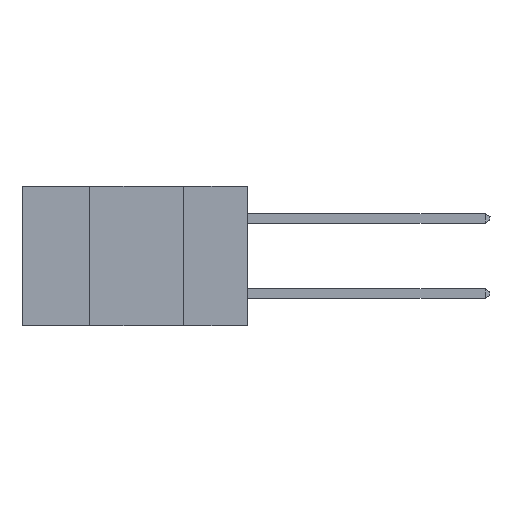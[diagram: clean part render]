
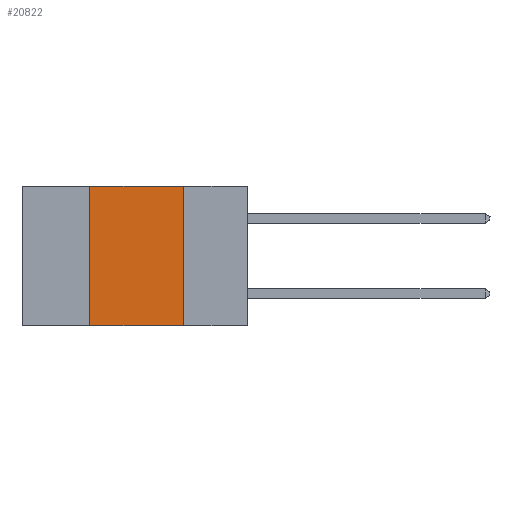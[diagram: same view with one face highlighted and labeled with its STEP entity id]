
A CAD part, left-side view. The second image highlights one B-rep face of the part: STEP entity #20822.
In plain terms, the highlighted planar face has unit normal (-1, 0, 0).
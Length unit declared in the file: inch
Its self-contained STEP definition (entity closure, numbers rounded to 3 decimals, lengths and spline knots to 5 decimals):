
#309 = VERTEX_POINT ( 'NONE', #16970 ) ;
#431 = LINE ( 'NONE', #25511, #8596 ) ;
#1226 = ORIENTED_EDGE ( 'NONE', *, *, #17684, .F. ) ;
#1428 = EDGE_LOOP ( 'NONE', ( #19657, #1226, #23308, #25156 ) ) ;
#2386 = DIRECTION ( 'NONE',  ( 0., -1., 0. ) ) ;
#2614 = VECTOR ( 'NONE', #24374, 39.37008 ) ;
#3199 = CARTESIAN_POINT ( 'NONE',  ( 0., 0.42, -0.37 ) ) ;
#4906 = LINE ( 'NONE', #6582, #13928 ) ;
#5536 = CARTESIAN_POINT ( 'NONE',  ( 0., 0.42, 0. ) ) ;
#6017 = VECTOR ( 'NONE', #7175, 39.37008 ) ;
#6582 = CARTESIAN_POINT ( 'NONE',  ( 0., 0.6, 0. ) ) ;
#6788 = VERTEX_POINT ( 'NONE', #23027 ) ;
#7175 = DIRECTION ( 'NONE',  ( 0., 0., -1. ) ) ;
#8028 = EDGE_CURVE ( 'NONE', #309, #6788, #13015, .T. ) ;
#8596 = VECTOR ( 'NONE', #2386, 39.37008 ) ;
#9742 = PLANE ( 'NONE',  #25899 ) ;
#12132 = EDGE_CURVE ( 'NONE', #26871, #19984, #13759, .T. ) ;
#13015 = LINE ( 'NONE', #15361, #6017 ) ;
#13416 = DIRECTION ( 'NONE',  ( 1., 0., 0. ) ) ;
#13759 = LINE ( 'NONE', #3199, #2614 ) ;
#13928 = VECTOR ( 'NONE', #19714, 39.37008 ) ;
#15361 = CARTESIAN_POINT ( 'NONE',  ( 0., 0.17, -0.37 ) ) ;
#15471 = FACE_OUTER_BOUND ( 'NONE', #1428, .T. ) ;
#16970 = CARTESIAN_POINT ( 'NONE',  ( 0., 0.17, 0. ) ) ;
#17684 = EDGE_CURVE ( 'NONE', #19984, #309, #4906, .T. ) ;
#18196 = CARTESIAN_POINT ( 'NONE',  ( 0., 0.6, 0. ) ) ;
#19657 = ORIENTED_EDGE ( 'NONE', *, *, #8028, .F. ) ;
#19714 = DIRECTION ( 'NONE',  ( 0., -1., 0. ) ) ;
#19737 = EDGE_CURVE ( 'NONE', #26871, #6788, #431, .T. ) ;
#19984 = VERTEX_POINT ( 'NONE', #5536 ) ;
#20453 = CARTESIAN_POINT ( 'NONE',  ( 0., 0.42, -0.37 ) ) ;
#20822 = ADVANCED_FACE ( 'NONE', ( #15471 ), #9742, .F. ) ;
#23027 = CARTESIAN_POINT ( 'NONE',  ( 0., 0.17, -0.37 ) ) ;
#23308 = ORIENTED_EDGE ( 'NONE', *, *, #12132, .F. ) ;
#24374 = DIRECTION ( 'NONE',  ( 0., 0., 1. ) ) ;
#25156 = ORIENTED_EDGE ( 'NONE', *, *, #19737, .T. ) ;
#25511 = CARTESIAN_POINT ( 'NONE',  ( 0., 0.6, -0.37 ) ) ;
#25715 = DIRECTION ( 'NONE',  ( 0., 0., -1. ) ) ;
#25899 = AXIS2_PLACEMENT_3D ( 'NONE', #18196, #13416, #25715 ) ;
#26871 = VERTEX_POINT ( 'NONE', #20453 ) ;
